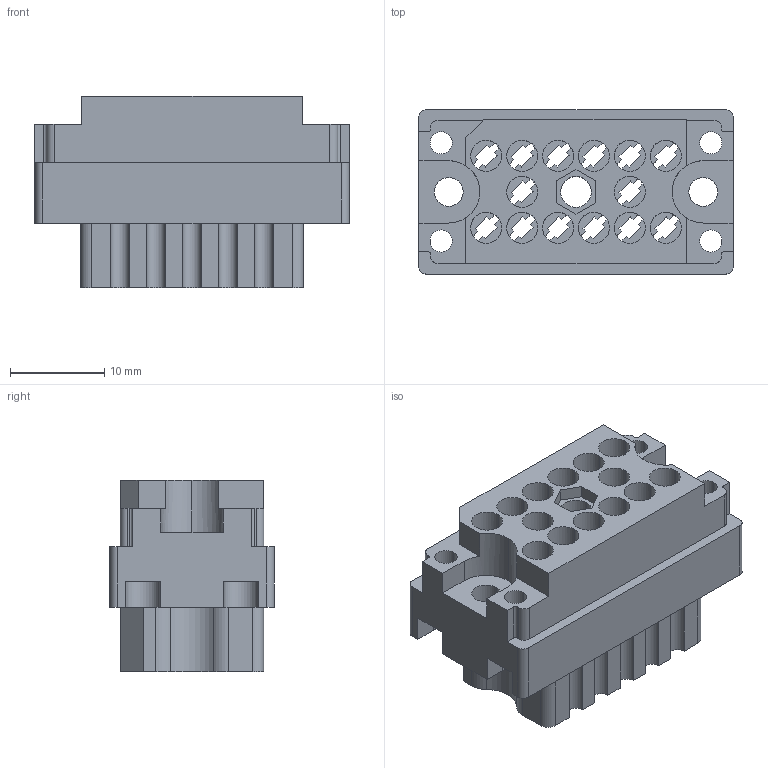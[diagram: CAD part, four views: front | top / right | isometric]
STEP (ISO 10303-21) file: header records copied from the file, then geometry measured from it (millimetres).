
FILE_DESCRIPTION (( 'STEP AP203' ), '1' );
FILE_NAME ('519-014-000-400.STEP', '2020-09-09T17:14:27', ( '' ), ( '' ), 'SwSTEP 2.0', 'SolidWorks 2020', '' );
FILE_SCHEMA (( 'CONFIG_CONTROL_DESIGN' ));
Length unit declared in the file: inch
Products named in the file (2): 519 Receptacle Insulator_014; 519-014-000-400
Assembly tree (1 placements, depth 2):
  519-014-000-400
    519 Receptacle Insulator_014
Bounding box: 33.32 x 17.42 x 20.27 mm (x, y, z)
Volume: 6062.6 mm3; surface area: 6883.4 mm2
Topology: 1 solids, 1 shells, 477 faces, 1391 edges, 926 vertices
Faces by surface type: plane 323, cylinder 152, cone 2
Entity records: 16081 total; most frequent: CARTESIAN_POINT 2798, ORIENTED_EDGE 2782, DIRECTION 2717, EDGE_CURVE 1391, LINE 1027, VECTOR 1027, VERTEX_POINT 926, AXIS2_PLACEMENT_3D 845
